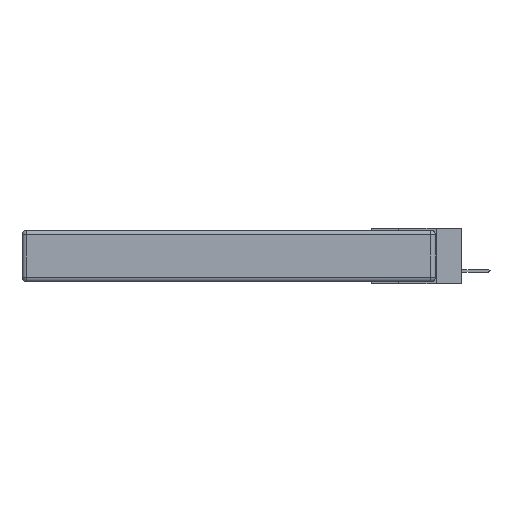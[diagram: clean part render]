
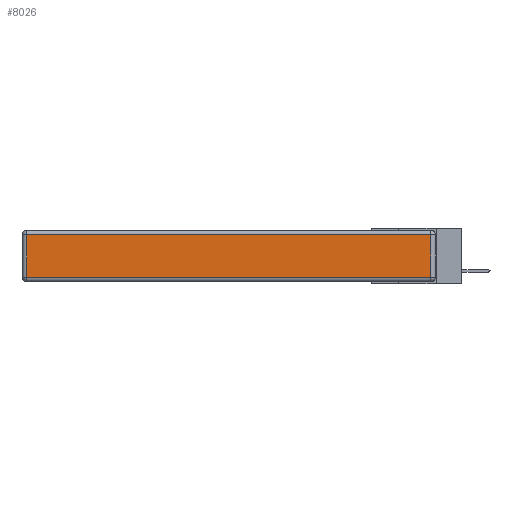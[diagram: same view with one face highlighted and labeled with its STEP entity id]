
A CAD part, left-side view. The second image highlights one B-rep face of the part: STEP entity #8026.
In plain terms, the highlighted planar face has unit normal (-1, 0, 0).
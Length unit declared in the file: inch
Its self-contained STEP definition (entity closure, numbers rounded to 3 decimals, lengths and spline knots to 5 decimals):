
#190 = DIRECTION ( 'NONE',  ( -1., 0., 0. ) ) ;
#361 = EDGE_LOOP ( 'NONE', ( #23410, #4954, #24398, #10919 ) ) ;
#581 = DIRECTION ( 'NONE',  ( 0., 0., 1. ) ) ;
#628 = LINE ( 'NONE', #19401, #14211 ) ;
#1157 = LINE ( 'NONE', #8460, #3297 ) ;
#1370 = AXIS2_PLACEMENT_3D ( 'NONE', #2165, #190, #6257 ) ;
#2165 = CARTESIAN_POINT ( 'NONE',  ( 0., 0., -0.343 ) ) ;
#3297 = VECTOR ( 'NONE', #581, 39.37008 ) ;
#4644 = CARTESIAN_POINT ( 'NONE',  ( 0., 0.03, -0.03 ) ) ;
#4668 = EDGE_CURVE ( 'NONE', #12144, #23458, #21582, .T. ) ;
#4695 = EDGE_CURVE ( 'NONE', #20602, #17035, #1157, .T. ) ;
#4954 = ORIENTED_EDGE ( 'NONE', *, *, #4695, .T. ) ;
#6257 = DIRECTION ( 'NONE',  ( 0., 0., 1. ) ) ;
#7656 = VECTOR ( 'NONE', #18200, 39.37008 ) ;
#8026 = ADVANCED_FACE ( 'NONE', ( #12364 ), #16049, .T. ) ;
#8460 = CARTESIAN_POINT ( 'NONE',  ( 0., 0.03, -0.343 ) ) ;
#8756 = DIRECTION ( 'NONE',  ( 0., 1., 0. ) ) ;
#9101 = CARTESIAN_POINT ( 'NONE',  ( 0., 0., -0.313 ) ) ;
#10857 = LINE ( 'NONE', #9101, #16747 ) ;
#10919 = ORIENTED_EDGE ( 'NONE', *, *, #4668, .T. ) ;
#12144 = VERTEX_POINT ( 'NONE', #14528 ) ;
#12364 = FACE_OUTER_BOUND ( 'NONE', #361, .T. ) ;
#12413 = EDGE_CURVE ( 'NONE', #17035, #12144, #628, .T. ) ;
#13955 = CARTESIAN_POINT ( 'NONE',  ( 0., 0.03, -0.313 ) ) ;
#14211 = VECTOR ( 'NONE', #8756, 39.37008 ) ;
#14528 = CARTESIAN_POINT ( 'NONE',  ( 0., 2.72, -0.03 ) ) ;
#16049 = PLANE ( 'NONE',  #1370 ) ;
#16747 = VECTOR ( 'NONE', #19034, 39.37008 ) ;
#17035 = VERTEX_POINT ( 'NONE', #4644 ) ;
#17801 = EDGE_CURVE ( 'NONE', #23458, #20602, #10857, .T. ) ;
#17964 = CARTESIAN_POINT ( 'NONE',  ( 0., 2.72, -0.313 ) ) ;
#18200 = DIRECTION ( 'NONE',  ( 0., 0., -1. ) ) ;
#19034 = DIRECTION ( 'NONE',  ( 0., -1., 0. ) ) ;
#19401 = CARTESIAN_POINT ( 'NONE',  ( 0., 2.75, -0.03 ) ) ;
#20270 = CARTESIAN_POINT ( 'NONE',  ( 0., 2.72, -0.343 ) ) ;
#20602 = VERTEX_POINT ( 'NONE', #13955 ) ;
#21582 = LINE ( 'NONE', #20270, #7656 ) ;
#23410 = ORIENTED_EDGE ( 'NONE', *, *, #17801, .T. ) ;
#23458 = VERTEX_POINT ( 'NONE', #17964 ) ;
#24398 = ORIENTED_EDGE ( 'NONE', *, *, #12413, .T. ) ;
